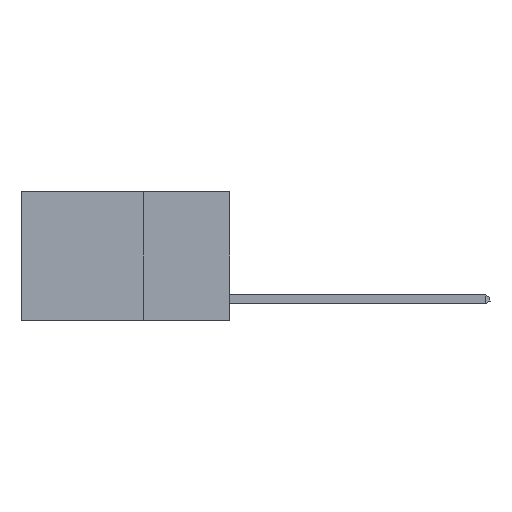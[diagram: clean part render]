
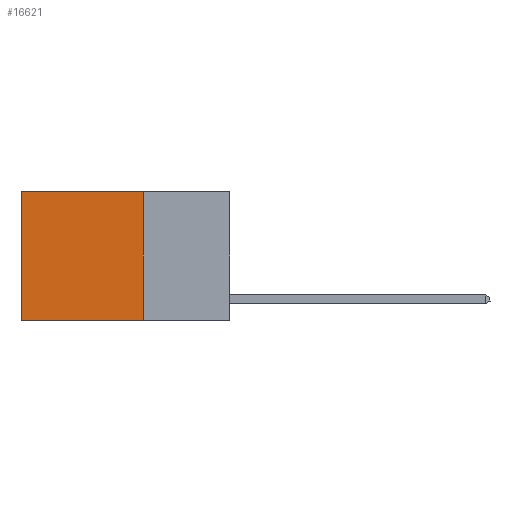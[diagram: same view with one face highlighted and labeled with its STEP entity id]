
A CAD part, left-side view. The second image highlights one B-rep face of the part: STEP entity #16621.
In plain terms, the highlighted planar face has unit normal (-1, 0, 0).
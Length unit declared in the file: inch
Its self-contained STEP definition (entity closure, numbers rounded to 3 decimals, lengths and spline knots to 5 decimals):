
#1445 = CARTESIAN_POINT ( 'NONE',  ( 0.2625, 0.6, 0. ) ) ;
#1918 = DIRECTION ( 'NONE',  ( 0., 1., 0. ) ) ;
#2565 = ORIENTED_EDGE ( 'NONE', *, *, #11375, .T. ) ;
#2713 = CARTESIAN_POINT ( 'NONE',  ( 0.2625, 0.25, 0. ) ) ;
#2753 = EDGE_LOOP ( 'NONE', ( #2565, #12732, #5722, #11287 ) ) ;
#2770 = PLANE ( 'NONE',  #3980 ) ;
#3422 = CARTESIAN_POINT ( 'NONE',  ( 0.2625, 0.25, -0.37 ) ) ;
#3980 = AXIS2_PLACEMENT_3D ( 'NONE', #2713, #13705, #6847 ) ;
#4295 = VERTEX_POINT ( 'NONE', #3422 ) ;
#4612 = VECTOR ( 'NONE', #1918, 39.37008 ) ;
#4657 = VERTEX_POINT ( 'NONE', #8167 ) ;
#4833 = LINE ( 'NONE', #6089, #4612 ) ;
#5722 = ORIENTED_EDGE ( 'NONE', *, *, #17262, .F. ) ;
#6089 = CARTESIAN_POINT ( 'NONE',  ( 0.2625, 0.25, -0.37 ) ) ;
#6485 = LINE ( 'NONE', #8152, #7531 ) ;
#6657 = DIRECTION ( 'NONE',  ( 0., 0., -1. ) ) ;
#6847 = DIRECTION ( 'NONE',  ( 0., 0., -1. ) ) ;
#7124 = CARTESIAN_POINT ( 'NONE',  ( 0.2625, 0.25, 0. ) ) ;
#7531 = VECTOR ( 'NONE', #6657, 39.37008 ) ;
#7793 = EDGE_CURVE ( 'NONE', #4657, #10535, #10852, .T. ) ;
#7820 = CARTESIAN_POINT ( 'NONE',  ( 0.2625, 0.6, -0.37 ) ) ;
#8051 = VERTEX_POINT ( 'NONE', #7820 ) ;
#8152 = CARTESIAN_POINT ( 'NONE',  ( 0.2625, 0.6, 0. ) ) ;
#8167 = CARTESIAN_POINT ( 'NONE',  ( 0.2625, 0.25, 0. ) ) ;
#9559 = EDGE_CURVE ( 'NONE', #4295, #8051, #4833, .T. ) ;
#10398 = VECTOR ( 'NONE', #16630, 39.37008 ) ;
#10535 = VERTEX_POINT ( 'NONE', #1445 ) ;
#10852 = LINE ( 'NONE', #15090, #10398 ) ;
#11287 = ORIENTED_EDGE ( 'NONE', *, *, #7793, .T. ) ;
#11375 = EDGE_CURVE ( 'NONE', #10535, #8051, #6485, .T. ) ;
#11430 = LINE ( 'NONE', #7124, #15529 ) ;
#12732 = ORIENTED_EDGE ( 'NONE', *, *, #9559, .F. ) ;
#13705 = DIRECTION ( 'NONE',  ( 1., 0., 0. ) ) ;
#14663 = FACE_OUTER_BOUND ( 'NONE', #2753, .T. ) ;
#15090 = CARTESIAN_POINT ( 'NONE',  ( 0.2625, 0.25, 0. ) ) ;
#15529 = VECTOR ( 'NONE', #16048, 39.37008 ) ;
#16048 = DIRECTION ( 'NONE',  ( 0., 0., -1. ) ) ;
#16621 = ADVANCED_FACE ( 'NONE', ( #14663 ), #2770, .F. ) ;
#16630 = DIRECTION ( 'NONE',  ( 0., 1., 0. ) ) ;
#17262 = EDGE_CURVE ( 'NONE', #4657, #4295, #11430, .T. ) ;
